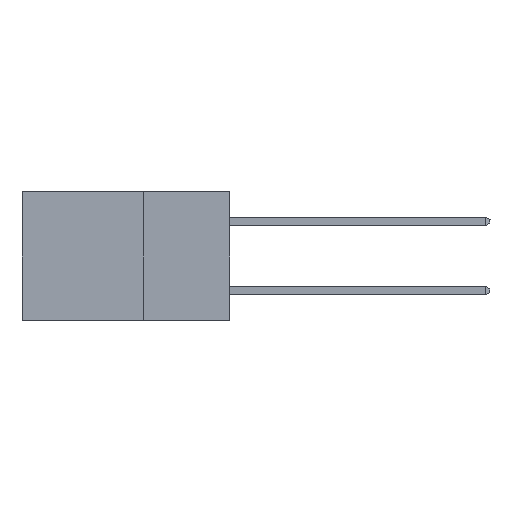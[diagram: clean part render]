
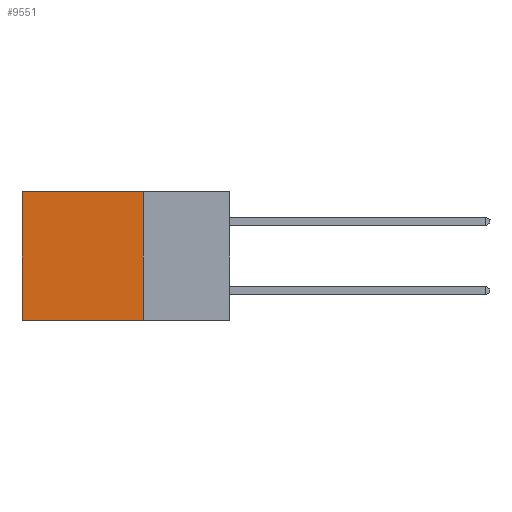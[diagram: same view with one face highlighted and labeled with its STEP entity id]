
A CAD part, left-side view. The second image highlights one B-rep face of the part: STEP entity #9551.
In plain terms, the highlighted planar face has unit normal (-1, 0, 0).
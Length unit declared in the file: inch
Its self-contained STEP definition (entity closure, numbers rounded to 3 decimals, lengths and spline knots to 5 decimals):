
#47 = VECTOR ( 'NONE', #18548, 39.37008 ) ;
#827 = AXIS2_PLACEMENT_3D ( 'NONE', #4401, #4106, #19562 ) ;
#1383 = VECTOR ( 'NONE', #7455, 39.37008 ) ;
#2675 = PLANE ( 'NONE',  #827 ) ;
#2739 = VERTEX_POINT ( 'NONE', #18398 ) ;
#3353 = DIRECTION ( 'NONE',  ( 0., 0., -1. ) ) ;
#3435 = VERTEX_POINT ( 'NONE', #18865 ) ;
#3678 = CARTESIAN_POINT ( 'NONE',  ( 0.2615, 0.25, -0.37 ) ) ;
#4106 = DIRECTION ( 'NONE',  ( 1., 0., 0. ) ) ;
#4208 = ORIENTED_EDGE ( 'NONE', *, *, #16180, .T. ) ;
#4401 = CARTESIAN_POINT ( 'NONE',  ( 0.2615, 0.25, -0.37 ) ) ;
#5068 = LINE ( 'NONE', #17235, #15193 ) ;
#6298 = CARTESIAN_POINT ( 'NONE',  ( 0.2615, 0.25, 0. ) ) ;
#6894 = DIRECTION ( 'NONE',  ( 0., 1., 0. ) ) ;
#7455 = DIRECTION ( 'NONE',  ( 0., 0., -1. ) ) ;
#7603 = VERTEX_POINT ( 'NONE', #11037 ) ;
#8367 = VERTEX_POINT ( 'NONE', #11802 ) ;
#9149 = CARTESIAN_POINT ( 'NONE',  ( 0.2615, 0.25, -0.37 ) ) ;
#9551 = ADVANCED_FACE ( 'NONE', ( #19660 ), #2675, .F. ) ;
#10555 = LINE ( 'NONE', #9149, #1383 ) ;
#11037 = CARTESIAN_POINT ( 'NONE',  ( 0.2615, 0.25, 0. ) ) ;
#11802 = CARTESIAN_POINT ( 'NONE',  ( 0.2615, 0.25, -0.37 ) ) ;
#12740 = ORIENTED_EDGE ( 'NONE', *, *, #18078, .T. ) ;
#12941 = ORIENTED_EDGE ( 'NONE', *, *, #19630, .F. ) ;
#13316 = VECTOR ( 'NONE', #6894, 39.37008 ) ;
#14525 = LINE ( 'NONE', #3678, #13316 ) ;
#15193 = VECTOR ( 'NONE', #3353, 39.37008 ) ;
#15229 = LINE ( 'NONE', #6298, #47 ) ;
#16180 = EDGE_CURVE ( 'NONE', #7603, #2739, #15229, .T. ) ;
#16492 = ORIENTED_EDGE ( 'NONE', *, *, #17156, .F. ) ;
#17156 = EDGE_CURVE ( 'NONE', #7603, #8367, #10555, .T. ) ;
#17235 = CARTESIAN_POINT ( 'NONE',  ( 0.2615, 0.6, -0.37 ) ) ;
#18078 = EDGE_CURVE ( 'NONE', #2739, #3435, #5068, .T. ) ;
#18398 = CARTESIAN_POINT ( 'NONE',  ( 0.2615, 0.6, 0. ) ) ;
#18548 = DIRECTION ( 'NONE',  ( 0., 1., 0. ) ) ;
#18820 = EDGE_LOOP ( 'NONE', ( #12740, #12941, #16492, #4208 ) ) ;
#18865 = CARTESIAN_POINT ( 'NONE',  ( 0.2615, 0.6, -0.37 ) ) ;
#19562 = DIRECTION ( 'NONE',  ( 0., 0., -1. ) ) ;
#19630 = EDGE_CURVE ( 'NONE', #8367, #3435, #14525, .T. ) ;
#19660 = FACE_OUTER_BOUND ( 'NONE', #18820, .T. ) ;
